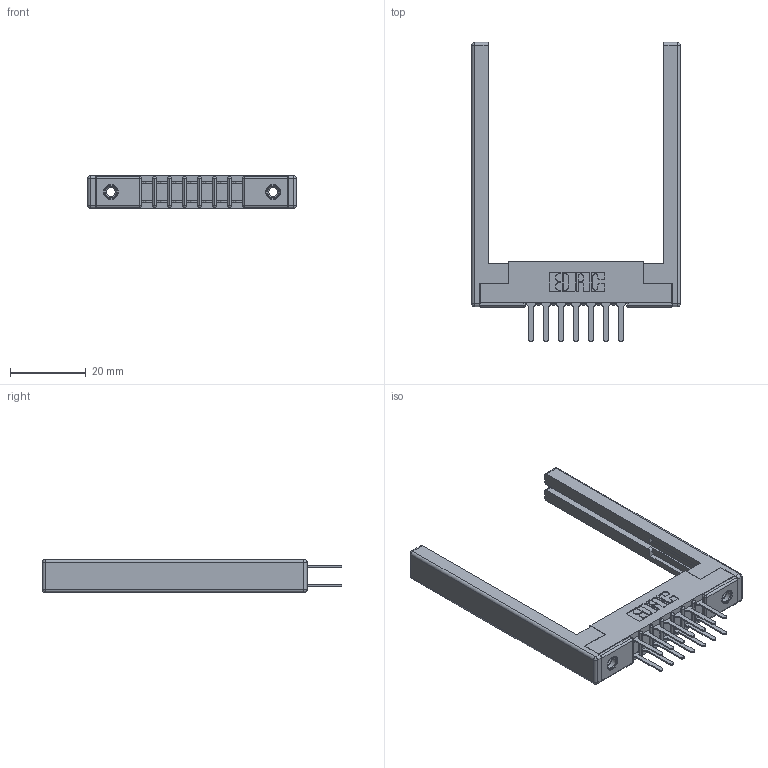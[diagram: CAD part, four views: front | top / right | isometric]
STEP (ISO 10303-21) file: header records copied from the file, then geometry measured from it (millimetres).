
FILE_DESCRIPTION (( 'STEP AP203' ), '1' );
FILE_NAME ('357-014-522-268.STEP', '2019-09-17T18:28:54', ( '' ), ( '' ), 'SwSTEP 2.0', 'SolidWorks 2016', '' );
FILE_SCHEMA (( 'CONFIG_CONTROL_DESIGN' ));
Length unit declared in the file: inch
Products named in the file (5): 307-220-068; 357-014-522-268; 345-250-001_345-250-001-102; 307 Part_.156 Dia Mounting Holes; 307-290-001_522
Assembly tree (19 placements, depth 2):
  357-014-522-268
    307 Part_.156 Dia Mounting Holes
    307-290-001_522  x14
    307-220-068  x2
    345-250-001_345-250-001-102  x2
Bounding box: 55.17 x 79.07 x 8.71 mm (x, y, z)
Volume: 8201.9 mm3; surface area: 9849.5 mm2
Topology: 19 solids, 19 shells, 924 faces, 2533 edges, 1626 vertices
Faces by surface type: plane 592, cylinder 292, sphere 24, cone 12, torus 4
Entity records: 13267 total; most frequent: CARTESIAN_POINT 2156, DIRECTION 2142, ORIENTED_EDGE 2124, EDGE_CURVE 1062, VECTOR 798, LINE 798, VERTEX_POINT 686, AXIS2_PLACEMENT_3D 672
